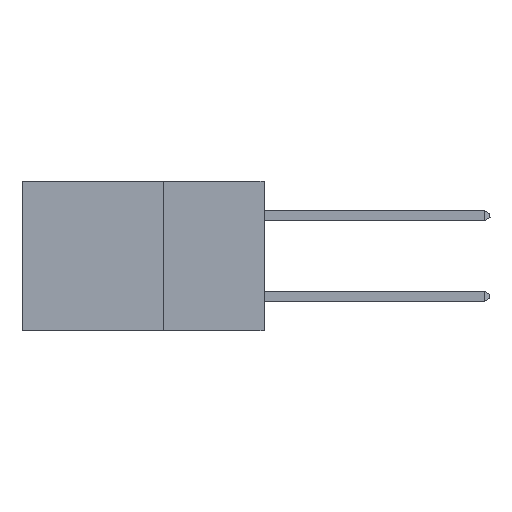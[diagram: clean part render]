
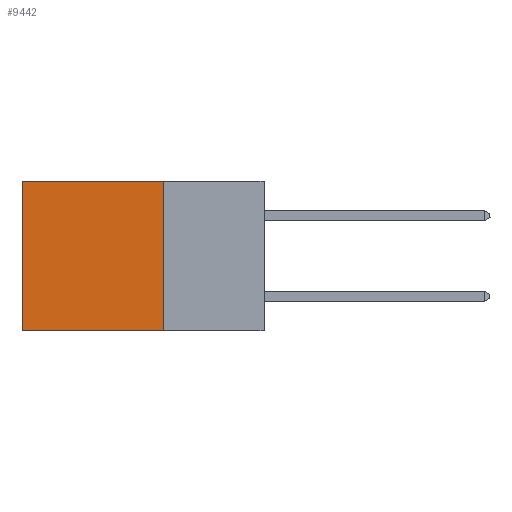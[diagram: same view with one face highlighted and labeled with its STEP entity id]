
A CAD part, left-side view. The second image highlights one B-rep face of the part: STEP entity #9442.
In plain terms, the highlighted planar face has unit normal (-1, 0, 0).
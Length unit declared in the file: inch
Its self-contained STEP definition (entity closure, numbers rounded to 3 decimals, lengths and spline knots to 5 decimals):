
#112 = CARTESIAN_POINT ( 'NONE',  ( 0.298, 0.25, 0. ) ) ;
#1015 = CARTESIAN_POINT ( 'NONE',  ( 0.298, 0.6, -0.37 ) ) ;
#1338 = CARTESIAN_POINT ( 'NONE',  ( 0.298, 0.6, 0. ) ) ;
#1531 = CARTESIAN_POINT ( 'NONE',  ( 0.298, 0.25, -0.37 ) ) ;
#1970 = PLANE ( 'NONE',  #17034 ) ;
#2850 = DIRECTION ( 'NONE',  ( 0., 1., 0. ) ) ;
#3389 = VECTOR ( 'NONE', #10515, 39.37008 ) ;
#3604 = EDGE_CURVE ( 'NONE', #5233, #7553, #6926, .T. ) ;
#4032 = VECTOR ( 'NONE', #4850, 39.37008 ) ;
#4463 = EDGE_CURVE ( 'NONE', #5717, #10756, #11868, .T. ) ;
#4850 = DIRECTION ( 'NONE',  ( 0., 1., 0. ) ) ;
#5233 = VERTEX_POINT ( 'NONE', #5511 ) ;
#5511 = CARTESIAN_POINT ( 'NONE',  ( 0.298, 0.25, -0.37 ) ) ;
#5717 = VERTEX_POINT ( 'NONE', #112 ) ;
#6472 = CARTESIAN_POINT ( 'NONE',  ( 0.298, 0.6, 0. ) ) ;
#6926 = LINE ( 'NONE', #1531, #12911 ) ;
#7553 = VERTEX_POINT ( 'NONE', #1015 ) ;
#9327 = CARTESIAN_POINT ( 'NONE',  ( 0.298, 0.25, 0. ) ) ;
#9442 = ADVANCED_FACE ( 'NONE', ( #12678 ), #1970, .F. ) ;
#9728 = DIRECTION ( 'NONE',  ( 0., 0., -1. ) ) ;
#10268 = EDGE_CURVE ( 'NONE', #10756, #7553, #14517, .T. ) ;
#10515 = DIRECTION ( 'NONE',  ( 0., 0., -1. ) ) ;
#10542 = ORIENTED_EDGE ( 'NONE', *, *, #15314, .F. ) ;
#10756 = VERTEX_POINT ( 'NONE', #6472 ) ;
#11255 = VECTOR ( 'NONE', #13099, 39.37008 ) ;
#11868 = LINE ( 'NONE', #12777, #4032 ) ;
#12210 = EDGE_LOOP ( 'NONE', ( #13903, #16256, #10542, #15740 ) ) ;
#12549 = DIRECTION ( 'NONE',  ( 1., 0., 0. ) ) ;
#12678 = FACE_OUTER_BOUND ( 'NONE', #12210, .T. ) ;
#12777 = CARTESIAN_POINT ( 'NONE',  ( 0.298, 0.25, 0. ) ) ;
#12911 = VECTOR ( 'NONE', #2850, 39.37008 ) ;
#13099 = DIRECTION ( 'NONE',  ( 0., 0., -1. ) ) ;
#13903 = ORIENTED_EDGE ( 'NONE', *, *, #10268, .T. ) ;
#14517 = LINE ( 'NONE', #1338, #3389 ) ;
#14826 = LINE ( 'NONE', #9327, #11255 ) ;
#15084 = CARTESIAN_POINT ( 'NONE',  ( 0.298, 0.25, 0. ) ) ;
#15314 = EDGE_CURVE ( 'NONE', #5717, #5233, #14826, .T. ) ;
#15740 = ORIENTED_EDGE ( 'NONE', *, *, #4463, .T. ) ;
#16256 = ORIENTED_EDGE ( 'NONE', *, *, #3604, .F. ) ;
#17034 = AXIS2_PLACEMENT_3D ( 'NONE', #15084, #12549, #9728 ) ;
